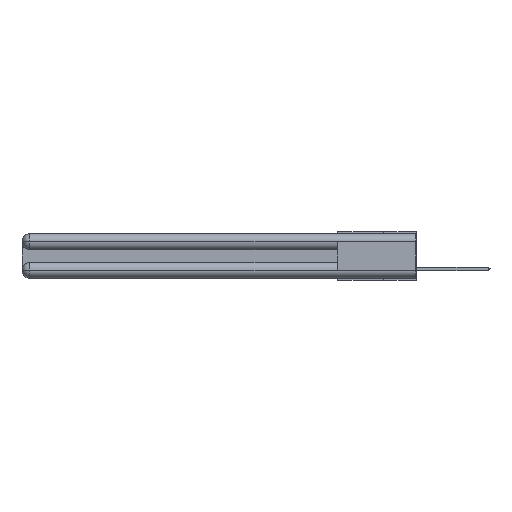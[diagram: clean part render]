
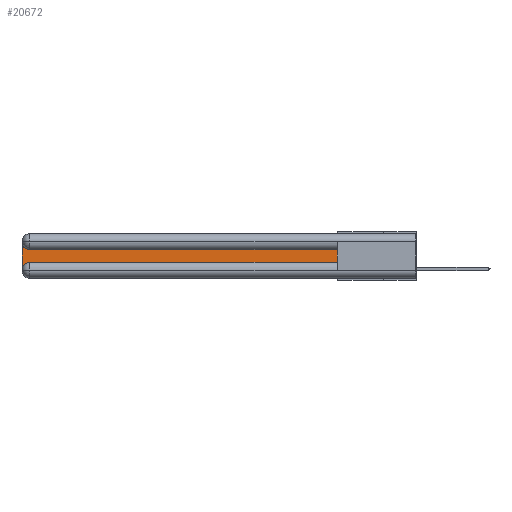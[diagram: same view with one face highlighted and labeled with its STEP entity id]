
A CAD part, left-side view. The second image highlights one B-rep face of the part: STEP entity #20672.
In plain terms, the highlighted planar face has unit normal (-1, 0, 0).
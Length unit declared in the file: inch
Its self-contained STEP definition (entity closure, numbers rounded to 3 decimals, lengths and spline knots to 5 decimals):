
#375 = AXIS2_PLACEMENT_3D ( 'NONE', #10664, #12703, #4394 ) ;
#654 = ORIENTED_EDGE ( 'NONE', *, *, #818, .T. ) ;
#818 = EDGE_CURVE ( 'NONE', #16952, #4458, #24430, .T. ) ;
#1577 = DIRECTION ( 'NONE',  ( 0., 0., 1. ) ) ;
#1830 = FACE_OUTER_BOUND ( 'NONE', #20149, .T. ) ;
#2027 = EDGE_CURVE ( 'NONE', #6136, #4869, #23380, .T. ) ;
#2489 = DIRECTION ( 'NONE',  ( 1., 0., 0. ) ) ;
#2941 = CARTESIAN_POINT ( 'NONE',  ( 0.075, 3., -0.0625 ) ) ;
#3343 = AXIS2_PLACEMENT_3D ( 'NONE', #24978, #12395, #8715 ) ;
#3540 = AXIS2_PLACEMENT_3D ( 'NONE', #25232, #2489, #15067 ) ;
#4394 = DIRECTION ( 'NONE',  ( 0., 0., -1. ) ) ;
#4458 = VERTEX_POINT ( 'NONE', #23058 ) ;
#4869 = VERTEX_POINT ( 'NONE', #18447 ) ;
#5008 = VECTOR ( 'NONE', #13750, 39.37008 ) ;
#5453 = CIRCLE ( 'NONE', #3343, 0.06 ) ;
#5592 = EDGE_CURVE ( 'NONE', #4869, #16952, #11339, .T. ) ;
#6136 = VERTEX_POINT ( 'NONE', #18223 ) ;
#6675 = VECTOR ( 'NONE', #8407, 39.37008 ) ;
#7884 = EDGE_CURVE ( 'NONE', #20899, #12569, #17503, .T. ) ;
#8407 = DIRECTION ( 'NONE',  ( 0., -1., 0. ) ) ;
#8715 = DIRECTION ( 'NONE',  ( 0., 0., -1. ) ) ;
#10664 = CARTESIAN_POINT ( 'NONE',  ( 0.075, 2.94, -0.2775 ) ) ;
#10700 = CARTESIAN_POINT ( 'NONE',  ( 0.075, 0.6, -0.1225 ) ) ;
#11339 = LINE ( 'NONE', #14125, #14673 ) ;
#12395 = DIRECTION ( 'NONE',  ( 1., 0., 0. ) ) ;
#12569 = VERTEX_POINT ( 'NONE', #15475 ) ;
#12703 = DIRECTION ( 'NONE',  ( 1., 0., 0. ) ) ;
#13750 = DIRECTION ( 'NONE',  ( 0., 0., -1. ) ) ;
#14125 = CARTESIAN_POINT ( 'NONE',  ( 0.075, 0.6, -0.2175 ) ) ;
#14673 = VECTOR ( 'NONE', #1577, 39.37008 ) ;
#14766 = CARTESIAN_POINT ( 'NONE',  ( 0.075, 0.6, -0.1225 ) ) ;
#14814 = ORIENTED_EDGE ( 'NONE', *, *, #7884, .T. ) ;
#15067 = DIRECTION ( 'NONE',  ( 0., 0., -1. ) ) ;
#15475 = CARTESIAN_POINT ( 'NONE',  ( 0.075, 3., -0.2775 ) ) ;
#16328 = ORIENTED_EDGE ( 'NONE', *, *, #5592, .T. ) ;
#16690 = CARTESIAN_POINT ( 'NONE',  ( 0.075, 0.6, -0.2175 ) ) ;
#16730 = DIRECTION ( 'NONE',  ( 0., 1., 0. ) ) ;
#16952 = VERTEX_POINT ( 'NONE', #14766 ) ;
#17465 = ORIENTED_EDGE ( 'NONE', *, *, #18280, .T. ) ;
#17503 = LINE ( 'NONE', #22300, #5008 ) ;
#18223 = CARTESIAN_POINT ( 'NONE',  ( 0.075, 2.94, -0.2175 ) ) ;
#18280 = EDGE_CURVE ( 'NONE', #4458, #20899, #5453, .T. ) ;
#18447 = CARTESIAN_POINT ( 'NONE',  ( 0.075, 0.6, -0.2175 ) ) ;
#18941 = PLANE ( 'NONE',  #3540 ) ;
#19075 = ORIENTED_EDGE ( 'NONE', *, *, #2027, .T. ) ;
#19475 = CIRCLE ( 'NONE', #375, 0.06 ) ;
#20149 = EDGE_LOOP ( 'NONE', ( #654, #17465, #14814, #22933, #19075, #16328 ) ) ;
#20672 = ADVANCED_FACE ( 'NONE', ( #1830 ), #18941, .F. ) ;
#20899 = VERTEX_POINT ( 'NONE', #2941 ) ;
#22158 = EDGE_CURVE ( 'NONE', #12569, #6136, #19475, .T. ) ;
#22300 = CARTESIAN_POINT ( 'NONE',  ( 0.075, 3., -0.2175 ) ) ;
#22933 = ORIENTED_EDGE ( 'NONE', *, *, #22158, .T. ) ;
#23058 = CARTESIAN_POINT ( 'NONE',  ( 0.075, 2.94, -0.1225 ) ) ;
#23380 = LINE ( 'NONE', #16690, #6675 ) ;
#24430 = LINE ( 'NONE', #10700, #26721 ) ;
#24978 = CARTESIAN_POINT ( 'NONE',  ( 0.075, 2.94, -0.0625 ) ) ;
#25232 = CARTESIAN_POINT ( 'NONE',  ( 0.075, 3., -0.1225 ) ) ;
#26721 = VECTOR ( 'NONE', #16730, 39.37008 ) ;
